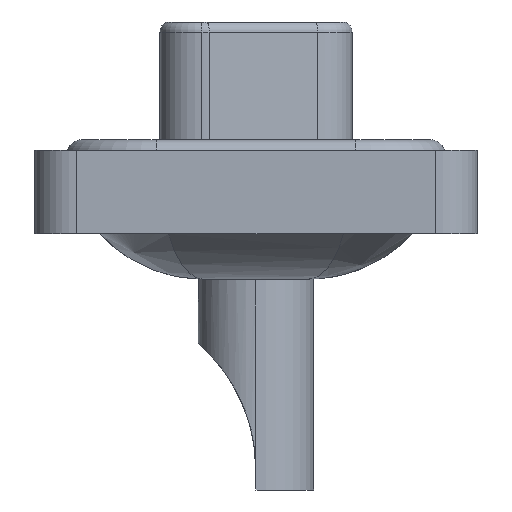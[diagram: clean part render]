
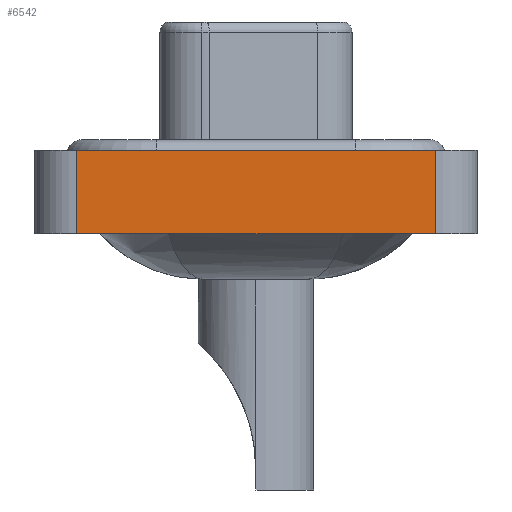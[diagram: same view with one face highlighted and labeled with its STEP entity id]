
A CAD part, left-side view. The second image highlights one B-rep face of the part: STEP entity #6542.
In plain terms, the highlighted planar face has unit normal (-1, 0, 0).
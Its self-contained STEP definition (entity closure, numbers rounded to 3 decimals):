
#484 = DIRECTION ( 'NONE',  ( 0., 0., 1. ) ) ;
#553 = EDGE_LOOP ( 'NONE', ( #3695, #808, #16520, #698 ) ) ;
#698 = ORIENTED_EDGE ( 'NONE', *, *, #8953, .T. ) ;
#808 = ORIENTED_EDGE ( 'NONE', *, *, #3970, .F. ) ;
#820 = PLANE ( 'NONE',  #14458 ) ;
#825 = LINE ( 'NONE', #11173, #2955 ) ;
#2484 = CARTESIAN_POINT ( 'NONE',  ( -7.3, -8.55, 0.4 ) ) ;
#2955 = VECTOR ( 'NONE', #4678, 1000. ) ;
#3280 = CARTESIAN_POINT ( 'NONE',  ( -7.3, -8.55, 0.4 ) ) ;
#3391 = DIRECTION ( 'NONE',  ( -1., 0., 0. ) ) ;
#3695 = ORIENTED_EDGE ( 'NONE', *, *, #14294, .T. ) ;
#3970 = EDGE_CURVE ( 'NONE', #4953, #9626, #8825, .T. ) ;
#4331 = LINE ( 'NONE', #9547, #8863 ) ;
#4678 = DIRECTION ( 'NONE',  ( 0., 0., 1. ) ) ;
#4953 = VERTEX_POINT ( 'NONE', #12426 ) ;
#5147 = DIRECTION ( 'NONE',  ( 0., -1., 0. ) ) ;
#6542 = ADVANCED_FACE ( 'NONE', ( #8693 ), #820, .T. ) ;
#6978 = EDGE_CURVE ( 'NONE', #9451, #4953, #4331, .T. ) ;
#7633 = VECTOR ( 'NONE', #5147, 1000. ) ;
#8693 = FACE_OUTER_BOUND ( 'NONE', #553, .T. ) ;
#8825 = LINE ( 'NONE', #2484, #7633 ) ;
#8863 = VECTOR ( 'NONE', #484, 1000. ) ;
#8953 = EDGE_CURVE ( 'NONE', #9451, #12865, #15518, .T. ) ;
#9451 = VERTEX_POINT ( 'NONE', #10124 ) ;
#9547 = CARTESIAN_POINT ( 'NONE',  ( -7.3, 8.55, -3.6 ) ) ;
#9626 = VERTEX_POINT ( 'NONE', #3280 ) ;
#10124 = CARTESIAN_POINT ( 'NONE',  ( -7.3, 8.55, -3.6 ) ) ;
#10396 = DIRECTION ( 'NONE',  ( 0., -1., 0. ) ) ;
#11173 = CARTESIAN_POINT ( 'NONE',  ( -7.3, -8.55, -3.6 ) ) ;
#11410 = DIRECTION ( 'NONE',  ( 0., 0., 1. ) ) ;
#11757 = CARTESIAN_POINT ( 'NONE',  ( -7.3, -8.55, -3.6 ) ) ;
#12426 = CARTESIAN_POINT ( 'NONE',  ( -7.3, 8.55, 0.4 ) ) ;
#12865 = VERTEX_POINT ( 'NONE', #15257 ) ;
#14294 = EDGE_CURVE ( 'NONE', #12865, #9626, #825, .T. ) ;
#14458 = AXIS2_PLACEMENT_3D ( 'NONE', #16293, #3391, #11410 ) ;
#15109 = VECTOR ( 'NONE', #10396, 1000. ) ;
#15257 = CARTESIAN_POINT ( 'NONE',  ( -7.3, -8.55, -3.6 ) ) ;
#15518 = LINE ( 'NONE', #11757, #15109 ) ;
#16293 = CARTESIAN_POINT ( 'NONE',  ( -7.3, -8.55, -3.6 ) ) ;
#16520 = ORIENTED_EDGE ( 'NONE', *, *, #6978, .F. ) ;
